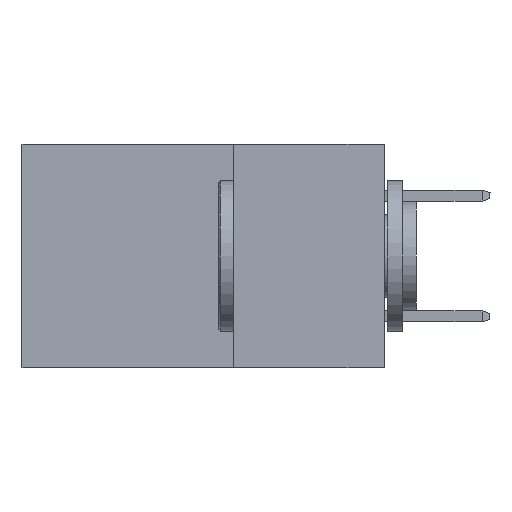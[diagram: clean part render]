
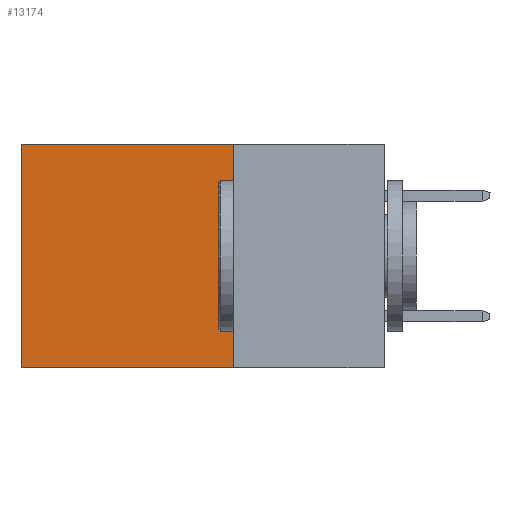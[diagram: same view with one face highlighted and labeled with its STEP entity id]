
A CAD part, left-side view. The second image highlights one B-rep face of the part: STEP entity #13174.
In plain terms, the highlighted planar face has unit normal (-1, 0, 0).
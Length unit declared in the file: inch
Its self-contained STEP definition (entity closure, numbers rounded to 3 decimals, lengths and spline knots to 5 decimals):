
#366 = AXIS2_PLACEMENT_3D ( 'NONE', #8262, #3246, #30540 ) ;
#1278 = DIRECTION ( 'NONE',  ( 0., 1., 0. ) ) ;
#3246 = DIRECTION ( 'NONE',  ( 1., 0., 0. ) ) ;
#3380 = VECTOR ( 'NONE', #15203, 39.37008 ) ;
#4047 = FACE_OUTER_BOUND ( 'NONE', #29970, .T. ) ;
#4932 = VECTOR ( 'NONE', #1278, 39.37008 ) ;
#6557 = VECTOR ( 'NONE', #25157, 39.37008 ) ;
#6690 = ORIENTED_EDGE ( 'NONE', *, *, #22197, .T. ) ;
#6966 = VERTEX_POINT ( 'NONE', #14233 ) ;
#8262 = CARTESIAN_POINT ( 'NONE',  ( 0.298, 0.25, 0. ) ) ;
#8638 = ORIENTED_EDGE ( 'NONE', *, *, #27088, .F. ) ;
#9839 = VERTEX_POINT ( 'NONE', #12933 ) ;
#9864 = CARTESIAN_POINT ( 'NONE',  ( 0.298, 0.25, 0. ) ) ;
#12768 = CARTESIAN_POINT ( 'NONE',  ( 0.298, 0.25, 0. ) ) ;
#12933 = CARTESIAN_POINT ( 'NONE',  ( 0.298, 0.6, 0. ) ) ;
#13174 = ADVANCED_FACE ( 'NONE', ( #4047 ), #24516, .F. ) ;
#14233 = CARTESIAN_POINT ( 'NONE',  ( 0.298, 0.25, -0.37 ) ) ;
#15203 = DIRECTION ( 'NONE',  ( 0., 0., -1. ) ) ;
#15274 = ORIENTED_EDGE ( 'NONE', *, *, #21464, .F. ) ;
#15546 = LINE ( 'NONE', #25391, #4932 ) ;
#16398 = LINE ( 'NONE', #17298, #6557 ) ;
#17298 = CARTESIAN_POINT ( 'NONE',  ( 0.298, 0.25, 0. ) ) ;
#18206 = VERTEX_POINT ( 'NONE', #9864 ) ;
#19155 = EDGE_CURVE ( 'NONE', #18206, #9839, #16398, .T. ) ;
#19874 = VERTEX_POINT ( 'NONE', #24162 ) ;
#21464 = EDGE_CURVE ( 'NONE', #6966, #19874, #15546, .T. ) ;
#22197 = EDGE_CURVE ( 'NONE', #9839, #19874, #23791, .T. ) ;
#23791 = LINE ( 'NONE', #28657, #29107 ) ;
#24162 = CARTESIAN_POINT ( 'NONE',  ( 0.298, 0.6, -0.37 ) ) ;
#24516 = PLANE ( 'NONE',  #366 ) ;
#25157 = DIRECTION ( 'NONE',  ( 0., 1., 0. ) ) ;
#25391 = CARTESIAN_POINT ( 'NONE',  ( 0.298, 0.25, -0.37 ) ) ;
#27088 = EDGE_CURVE ( 'NONE', #18206, #6966, #27577, .T. ) ;
#27577 = LINE ( 'NONE', #12768, #3380 ) ;
#28589 = ORIENTED_EDGE ( 'NONE', *, *, #19155, .T. ) ;
#28657 = CARTESIAN_POINT ( 'NONE',  ( 0.298, 0.6, 0. ) ) ;
#29107 = VECTOR ( 'NONE', #31027, 39.37008 ) ;
#29970 = EDGE_LOOP ( 'NONE', ( #6690, #15274, #8638, #28589 ) ) ;
#30540 = DIRECTION ( 'NONE',  ( 0., 0., -1. ) ) ;
#31027 = DIRECTION ( 'NONE',  ( 0., 0., -1. ) ) ;
